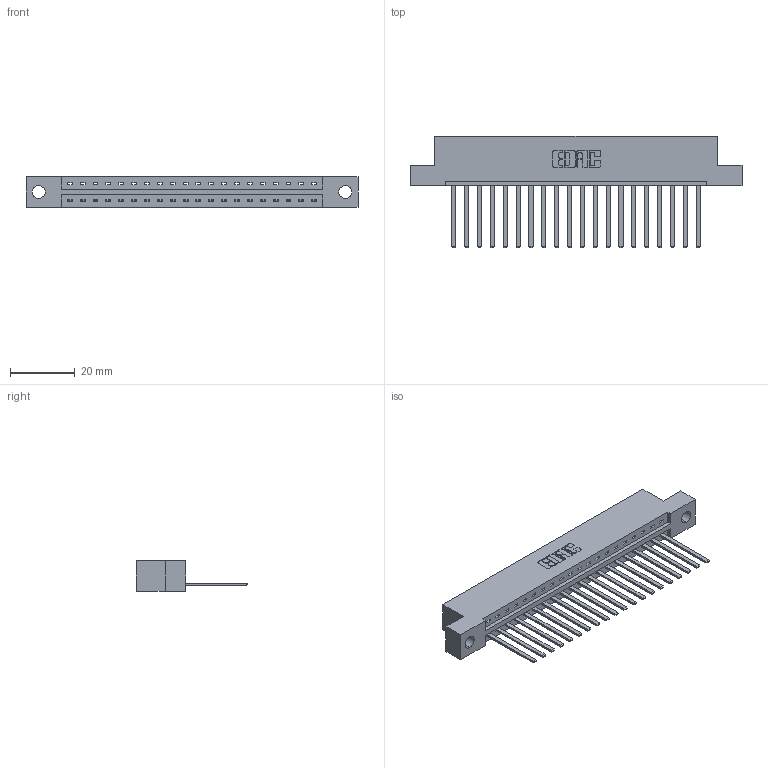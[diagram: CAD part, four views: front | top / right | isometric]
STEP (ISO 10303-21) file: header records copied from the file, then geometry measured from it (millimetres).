
FILE_DESCRIPTION (( 'STEP AP203' ), '1' );
FILE_NAME ('337-020-544-104.STEP', '2019-09-28T23:26:25', ( '' ), ( '' ), 'SwSTEP 2.0', 'SolidWorks 2016', '' );
FILE_SCHEMA (( 'CONFIG_CONTROL_DESIGN' ));
Length unit declared in the file: inch
Products named in the file (3): 345-292-001_345-293-144; 337 Part_Flush Mounting Lugs - 0.156 Dia-TH; 337-020-544-104
Assembly tree (21 placements, depth 2):
  337-020-544-104
    337 Part_Flush Mounting Lugs - 0.156 Dia-TH
    345-292-001_345-293-144  x20
Bounding box: 102.26 x 34.3 x 9.4 mm (x, y, z)
Volume: 10496.7 mm3; surface area: 11281.9 mm2
Topology: 21 solids, 21 shells, 1234 faces, 3711 edges, 2446 vertices
Faces by surface type: plane 910, cylinder 324
Entity records: 17531 total; most frequent: CARTESIAN_POINT 3058, ORIENTED_EDGE 3014, DIRECTION 2615, EDGE_CURVE 1507, VECTOR 1383, LINE 1383, VERTEX_POINT 1002, AXIS2_PLACEMENT_3D 616
